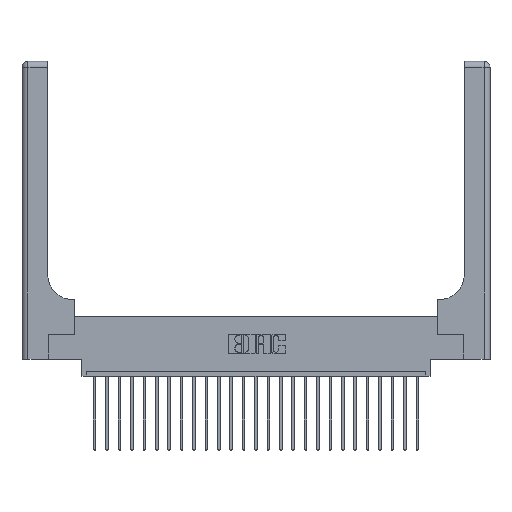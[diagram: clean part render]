
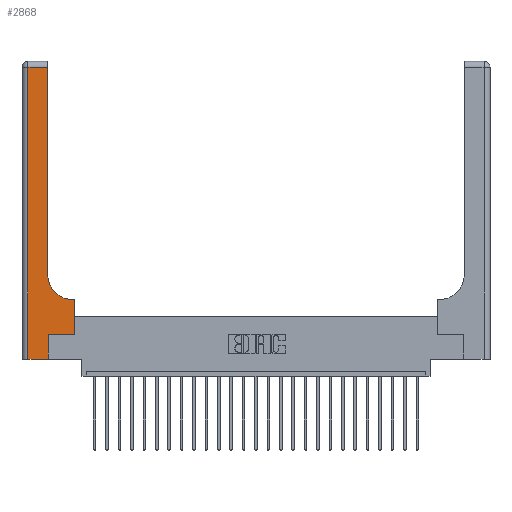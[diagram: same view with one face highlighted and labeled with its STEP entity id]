
A CAD part, top view. The second image highlights one B-rep face of the part: STEP entity #2868.
In plain terms, the highlighted planar face has unit normal (0, 0, 1).
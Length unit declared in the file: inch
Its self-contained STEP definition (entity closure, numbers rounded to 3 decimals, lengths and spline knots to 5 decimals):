
#279 = LINE ( 'NONE', #24383, #3233 ) ;
#378 = LINE ( 'NONE', #7968, #19199 ) ;
#720 = EDGE_CURVE ( 'NONE', #23463, #9346, #13376, .T. ) ;
#736 = VECTOR ( 'NONE', #2965, 39.37008 ) ;
#945 = ORIENTED_EDGE ( 'NONE', *, *, #13776, .T. ) ;
#1044 = ORIENTED_EDGE ( 'NONE', *, *, #17542, .T. ) ;
#1340 = VERTEX_POINT ( 'NONE', #13925 ) ;
#1560 = EDGE_LOOP ( 'NONE', ( #17440, #18285, #20501, #14480, #5192, #4167, #7769, #945, #1044 ) ) ;
#1935 = CARTESIAN_POINT ( 'NONE',  ( 0.26, 3., 0.37 ) ) ;
#2051 = EDGE_CURVE ( 'NONE', #16891, #1340, #20844, .T. ) ;
#2452 = EDGE_CURVE ( 'NONE', #9346, #16890, #279, .T. ) ;
#2868 = ADVANCED_FACE ( 'NONE', ( #11440 ), #17286, .F. ) ;
#2965 = DIRECTION ( 'NONE',  ( 0., -1., 0. ) ) ;
#3233 = VECTOR ( 'NONE', #3748, 39.37008 ) ;
#3260 = CARTESIAN_POINT ( 'NONE',  ( 0.51, 0.85, 0.37 ) ) ;
#3699 = AXIS2_PLACEMENT_3D ( 'NONE', #3260, #22032, #18446 ) ;
#3748 = DIRECTION ( 'NONE',  ( 1., 0., 0. ) ) ;
#4167 = ORIENTED_EDGE ( 'NONE', *, *, #8268, .T. ) ;
#4300 = CARTESIAN_POINT ( 'NONE',  ( 0.528, 0.25, 0.37 ) ) ;
#4592 = VERTEX_POINT ( 'NONE', #18864 ) ;
#5171 = CARTESIAN_POINT ( 'NONE',  ( 0.528, 0.25, 0.37 ) ) ;
#5192 = ORIENTED_EDGE ( 'NONE', *, *, #19255, .T. ) ;
#5226 = VECTOR ( 'NONE', #15012, 39.37008 ) ;
#5443 = CARTESIAN_POINT ( 'NONE',  ( 0.06, 0., 0.37 ) ) ;
#5484 = VERTEX_POINT ( 'NONE', #8294 ) ;
#5725 = DIRECTION ( 'NONE',  ( -1., 0., 0. ) ) ;
#7672 = CARTESIAN_POINT ( 'NONE',  ( 0.06, 2.94, 0.37 ) ) ;
#7719 = DIRECTION ( 'NONE',  ( 0., 0., -1. ) ) ;
#7769 = ORIENTED_EDGE ( 'NONE', *, *, #14562, .T. ) ;
#7968 = CARTESIAN_POINT ( 'NONE',  ( 0.265, 0., 0.37 ) ) ;
#8268 = EDGE_CURVE ( 'NONE', #5484, #15693, #16468, .T. ) ;
#8294 = CARTESIAN_POINT ( 'NONE',  ( 0.265, 0.25, 0.37 ) ) ;
#9202 = LINE ( 'NONE', #16670, #18851 ) ;
#9346 = VERTEX_POINT ( 'NONE', #5443 ) ;
#11440 = FACE_OUTER_BOUND ( 'NONE', #1560, .T. ) ;
#12003 = LINE ( 'NONE', #4300, #21963 ) ;
#12546 = VERTEX_POINT ( 'NONE', #17256 ) ;
#13376 = LINE ( 'NONE', #20833, #736 ) ;
#13776 = EDGE_CURVE ( 'NONE', #12546, #4592, #16545, .T. ) ;
#13925 = CARTESIAN_POINT ( 'NONE',  ( 0.26, 2.94, 0.37 ) ) ;
#14020 = CIRCLE ( 'NONE', #3699, 0.25 ) ;
#14477 = DIRECTION ( 'NONE',  ( 1., 0., 0. ) ) ;
#14480 = ORIENTED_EDGE ( 'NONE', *, *, #2452, .T. ) ;
#14562 = EDGE_CURVE ( 'NONE', #15693, #12546, #12003, .T. ) ;
#14984 = EDGE_CURVE ( 'NONE', #1340, #23463, #9202, .T. ) ;
#15012 = DIRECTION ( 'NONE',  ( 0., 1., 0. ) ) ;
#15045 = CARTESIAN_POINT ( 'NONE',  ( 0.265, 0., 0.37 ) ) ;
#15693 = VERTEX_POINT ( 'NONE', #5171 ) ;
#16423 = VECTOR ( 'NONE', #22112, 39.37008 ) ;
#16468 = LINE ( 'NONE', #24019, #18160 ) ;
#16545 = LINE ( 'NONE', #21985, #16423 ) ;
#16670 = CARTESIAN_POINT ( 'NONE',  ( 0., 2.94, 0.37 ) ) ;
#16890 = VERTEX_POINT ( 'NONE', #15045 ) ;
#16891 = VERTEX_POINT ( 'NONE', #22380 ) ;
#17256 = CARTESIAN_POINT ( 'NONE',  ( 0.528, 0.6, 0.37 ) ) ;
#17286 = PLANE ( 'NONE',  #23881 ) ;
#17440 = ORIENTED_EDGE ( 'NONE', *, *, #2051, .T. ) ;
#17542 = EDGE_CURVE ( 'NONE', #4592, #16891, #14020, .T. ) ;
#18160 = VECTOR ( 'NONE', #14477, 39.37008 ) ;
#18285 = ORIENTED_EDGE ( 'NONE', *, *, #14984, .T. ) ;
#18400 = DIRECTION ( 'NONE',  ( -1., 0., 0. ) ) ;
#18446 = DIRECTION ( 'NONE',  ( 1., 0., 0. ) ) ;
#18851 = VECTOR ( 'NONE', #18400, 39.37008 ) ;
#18864 = CARTESIAN_POINT ( 'NONE',  ( 0.51, 0.6, 0.37 ) ) ;
#19199 = VECTOR ( 'NONE', #21366, 39.37008 ) ;
#19255 = EDGE_CURVE ( 'NONE', #16890, #5484, #378, .T. ) ;
#20501 = ORIENTED_EDGE ( 'NONE', *, *, #720, .T. ) ;
#20833 = CARTESIAN_POINT ( 'NONE',  ( 0.06, 3., 0.37 ) ) ;
#20844 = LINE ( 'NONE', #1935, #5226 ) ;
#21366 = DIRECTION ( 'NONE',  ( 0., 1., 0. ) ) ;
#21427 = DIRECTION ( 'NONE',  ( 0., 1., 0. ) ) ;
#21963 = VECTOR ( 'NONE', #21427, 39.37008 ) ;
#21985 = CARTESIAN_POINT ( 'NONE',  ( 0.26, 0.6, 0.37 ) ) ;
#22032 = DIRECTION ( 'NONE',  ( 0., 0., -1. ) ) ;
#22112 = DIRECTION ( 'NONE',  ( -1., 0., 0. ) ) ;
#22380 = CARTESIAN_POINT ( 'NONE',  ( 0.26, 0.85, 0.37 ) ) ;
#22616 = CARTESIAN_POINT ( 'NONE',  ( 0., 3., 0.37 ) ) ;
#23463 = VERTEX_POINT ( 'NONE', #7672 ) ;
#23881 = AXIS2_PLACEMENT_3D ( 'NONE', #22616, #7719, #5725 ) ;
#24019 = CARTESIAN_POINT ( 'NONE',  ( 0.265, 0.25, 0.37 ) ) ;
#24383 = CARTESIAN_POINT ( 'NONE',  ( 0., 0., 0.37 ) ) ;
